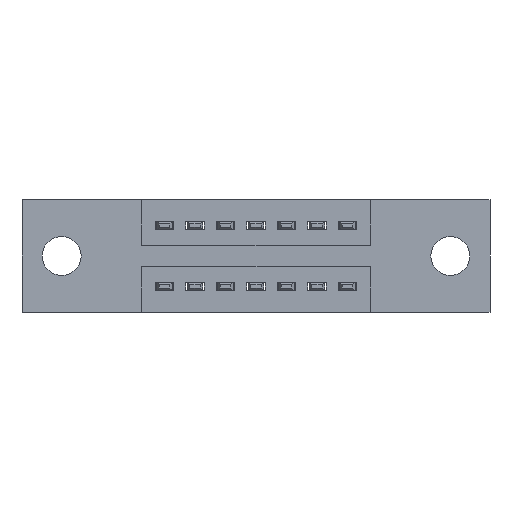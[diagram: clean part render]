
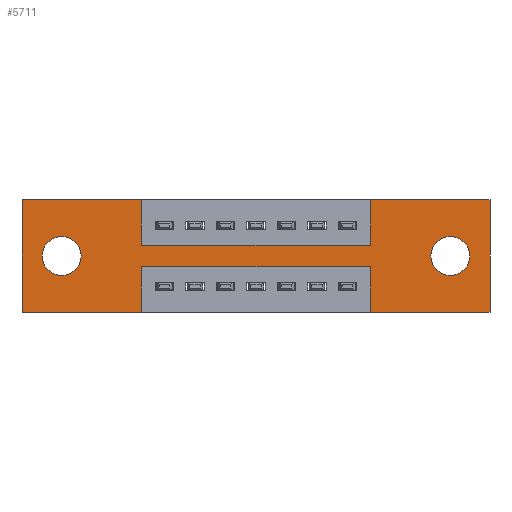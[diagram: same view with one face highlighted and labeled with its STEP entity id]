
A CAD part, front view. The second image highlights one B-rep face of the part: STEP entity #5711.
In plain terms, the highlighted planar face has unit normal (0, -1, 0).
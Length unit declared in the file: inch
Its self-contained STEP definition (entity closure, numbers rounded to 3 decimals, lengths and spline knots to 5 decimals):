
#54 = EDGE_CURVE ( 'NONE', #3700, #504, #7394, .T. ) ;
#79 = FACE_BOUND ( 'NONE', #6744, .T. ) ;
#148 = VECTOR ( 'NONE', #2319, 39.37008 ) ;
#348 = LINE ( 'NONE', #2535, #2153 ) ;
#473 = VERTEX_POINT ( 'NONE', #7672 ) ;
#504 = VERTEX_POINT ( 'NONE', #2349 ) ;
#685 = EDGE_CURVE ( 'NONE', #8767, #1796, #7384, .T. ) ;
#791 = DIRECTION ( 'NONE',  ( 1., 0., 0. ) ) ;
#833 = CIRCLE ( 'NONE', #9277, 0.064 ) ;
#880 = CIRCLE ( 'NONE', #2902, 0.064 ) ;
#932 = FACE_OUTER_BOUND ( 'NONE', #9668, .T. ) ;
#947 = CARTESIAN_POINT ( 'NONE',  ( 1.405, 0., -0.185 ) ) ;
#966 = DIRECTION ( 'NONE',  ( -1., 0., 0. ) ) ;
#981 = DIRECTION ( 'NONE',  ( 0., 1., 0. ) ) ;
#1031 = EDGE_CURVE ( 'NONE', #4648, #4432, #4263, .T. ) ;
#1047 = LINE ( 'NONE', #3530, #5956 ) ;
#1112 = LINE ( 'NONE', #1610, #9343 ) ;
#1265 = CARTESIAN_POINT ( 'NONE',  ( 0., 0., -0.37 ) ) ;
#1318 = AXIS2_PLACEMENT_3D ( 'NONE', #8120, #7399, #2808 ) ;
#1350 = CARTESIAN_POINT ( 'NONE',  ( 1.405, 0., -0.249 ) ) ;
#1355 = EDGE_CURVE ( 'NONE', #1935, #1695, #4728, .T. ) ;
#1462 = LINE ( 'NONE', #9288, #2197 ) ;
#1490 = VERTEX_POINT ( 'NONE', #4366 ) ;
#1610 = CARTESIAN_POINT ( 'NONE',  ( 1.1425, 0., -0.37 ) ) ;
#1665 = DIRECTION ( 'NONE',  ( 1., 0., 0. ) ) ;
#1684 = VERTEX_POINT ( 'NONE', #8054 ) ;
#1695 = VERTEX_POINT ( 'NONE', #8088 ) ;
#1796 = VERTEX_POINT ( 'NONE', #2870 ) ;
#1935 = VERTEX_POINT ( 'NONE', #3185 ) ;
#1985 = EDGE_CURVE ( 'NONE', #1796, #1935, #1112, .T. ) ;
#2035 = DIRECTION ( 'NONE',  ( 0., 0., -1. ) ) ;
#2130 = FACE_BOUND ( 'NONE', #6318, .T. ) ;
#2153 = VECTOR ( 'NONE', #4947, 39.37008 ) ;
#2197 = VECTOR ( 'NONE', #791, 39.37008 ) ;
#2272 = DIRECTION ( 'NONE',  ( 0., 1., 0. ) ) ;
#2319 = DIRECTION ( 'NONE',  ( 0., 0., 1. ) ) ;
#2349 = CARTESIAN_POINT ( 'NONE',  ( 1.405, 0., -0.121 ) ) ;
#2425 = DIRECTION ( 'NONE',  ( 0., 0., -1. ) ) ;
#2471 = CARTESIAN_POINT ( 'NONE',  ( 0.13, 0., -0.185 ) ) ;
#2478 = ORIENTED_EDGE ( 'NONE', *, *, #1985, .F. ) ;
#2535 = CARTESIAN_POINT ( 'NONE',  ( 1.1425, 0., 0. ) ) ;
#2577 = ORIENTED_EDGE ( 'NONE', *, *, #54, .T. ) ;
#2730 = DIRECTION ( 'NONE',  ( 0., 1., 0. ) ) ;
#2769 = VECTOR ( 'NONE', #2035, 39.37008 ) ;
#2808 = DIRECTION ( 'NONE',  ( 0., 0., -1. ) ) ;
#2814 = VECTOR ( 'NONE', #6021, 39.37008 ) ;
#2870 = CARTESIAN_POINT ( 'NONE',  ( 1.1425, 0., -0.37 ) ) ;
#2902 = AXIS2_PLACEMENT_3D ( 'NONE', #7319, #2730, #8102 ) ;
#2945 = CARTESIAN_POINT ( 'NONE',  ( 0.3925, 0., 0. ) ) ;
#2947 = LINE ( 'NONE', #1265, #6787 ) ;
#3185 = CARTESIAN_POINT ( 'NONE',  ( 1.1425, 0., -0.22 ) ) ;
#3530 = CARTESIAN_POINT ( 'NONE',  ( 0., 0., 0. ) ) ;
#3567 = EDGE_CURVE ( 'NONE', #473, #8945, #833, .T. ) ;
#3586 = VERTEX_POINT ( 'NONE', #5769 ) ;
#3681 = ORIENTED_EDGE ( 'NONE', *, *, #5395, .F. ) ;
#3700 = VERTEX_POINT ( 'NONE', #1350 ) ;
#3935 = CARTESIAN_POINT ( 'NONE',  ( 0.3925, 0., -0.22 ) ) ;
#4042 = CARTESIAN_POINT ( 'NONE',  ( 0., 0., -0.37 ) ) ;
#4152 = EDGE_CURVE ( 'NONE', #3586, #4873, #348, .T. ) ;
#4258 = CARTESIAN_POINT ( 'NONE',  ( 1.535, 0., 0. ) ) ;
#4263 = LINE ( 'NONE', #9400, #148 ) ;
#4309 = VECTOR ( 'NONE', #1665, 39.37008 ) ;
#4366 = CARTESIAN_POINT ( 'NONE',  ( 0.3925, 0., -0.15 ) ) ;
#4381 = EDGE_CURVE ( 'NONE', #1695, #8829, #4810, .T. ) ;
#4431 = CARTESIAN_POINT ( 'NONE',  ( 0., 0., -0.37 ) ) ;
#4432 = VERTEX_POINT ( 'NONE', #7391 ) ;
#4583 = ORIENTED_EDGE ( 'NONE', *, *, #4152, .F. ) ;
#4648 = VERTEX_POINT ( 'NONE', #4431 ) ;
#4728 = LINE ( 'NONE', #3935, #8218 ) ;
#4747 = CARTESIAN_POINT ( 'NONE',  ( 0.3925, 0., -0.15 ) ) ;
#4810 = LINE ( 'NONE', #5676, #2769 ) ;
#4873 = VERTEX_POINT ( 'NONE', #8543 ) ;
#4947 = DIRECTION ( 'NONE',  ( 0., 0., 1. ) ) ;
#5012 = ORIENTED_EDGE ( 'NONE', *, *, #9839, .T. ) ;
#5086 = CARTESIAN_POINT ( 'NONE',  ( 0.3925, 0., -0.37 ) ) ;
#5132 = ORIENTED_EDGE ( 'NONE', *, *, #1031, .F. ) ;
#5139 = AXIS2_PLACEMENT_3D ( 'NONE', #5803, #2272, #5225 ) ;
#5218 = CARTESIAN_POINT ( 'NONE',  ( 1.535, 0., 0. ) ) ;
#5225 = DIRECTION ( 'NONE',  ( 0., 0., -1. ) ) ;
#5279 = ORIENTED_EDGE ( 'NONE', *, *, #4381, .F. ) ;
#5284 = ORIENTED_EDGE ( 'NONE', *, *, #6078, .F. ) ;
#5395 = EDGE_CURVE ( 'NONE', #1490, #3586, #8045, .T. ) ;
#5551 = VERTEX_POINT ( 'NONE', #4258 ) ;
#5676 = CARTESIAN_POINT ( 'NONE',  ( 0.3925, 0., -0.37 ) ) ;
#5711 = ADVANCED_FACE ( 'NONE', ( #2130, #79, #932 ), #5836, .T. ) ;
#5769 = CARTESIAN_POINT ( 'NONE',  ( 1.1425, 0., -0.15 ) ) ;
#5803 = CARTESIAN_POINT ( 'NONE',  ( 1.405, 0., -0.185 ) ) ;
#5836 = PLANE ( 'NONE',  #1318 ) ;
#5927 = DIRECTION ( 'NONE',  ( 0., 0., -1. ) ) ;
#5956 = VECTOR ( 'NONE', #9735, 39.37008 ) ;
#5990 = ORIENTED_EDGE ( 'NONE', *, *, #3567, .T. ) ;
#6021 = DIRECTION ( 'NONE',  ( 0., 0., -1. ) ) ;
#6078 = EDGE_CURVE ( 'NONE', #4873, #5551, #1047, .T. ) ;
#6120 = ORIENTED_EDGE ( 'NONE', *, *, #8074, .F. ) ;
#6236 = ORIENTED_EDGE ( 'NONE', *, *, #6897, .F. ) ;
#6318 = EDGE_LOOP ( 'NONE', ( #9372, #2577 ) ) ;
#6438 = CARTESIAN_POINT ( 'NONE',  ( 1.535, 0., -0.37 ) ) ;
#6656 = EDGE_CURVE ( 'NONE', #504, #3700, #8640, .T. ) ;
#6744 = EDGE_LOOP ( 'NONE', ( #5012, #5990 ) ) ;
#6787 = VECTOR ( 'NONE', #7158, 39.37008 ) ;
#6856 = DIRECTION ( 'NONE',  ( 0., 0., 1. ) ) ;
#6897 = EDGE_CURVE ( 'NONE', #8829, #4648, #2947, .T. ) ;
#7022 = DIRECTION ( 'NONE',  ( -1., 0., 0. ) ) ;
#7158 = DIRECTION ( 'NONE',  ( -1., 0., 0. ) ) ;
#7276 = VECTOR ( 'NONE', #966, 39.37008 ) ;
#7319 = CARTESIAN_POINT ( 'NONE',  ( 0.13, 0., -0.185 ) ) ;
#7384 = LINE ( 'NONE', #4042, #7276 ) ;
#7391 = CARTESIAN_POINT ( 'NONE',  ( 0., 0., 0. ) ) ;
#7394 = CIRCLE ( 'NONE', #5139, 0.064 ) ;
#7399 = DIRECTION ( 'NONE',  ( 0., -1., 0. ) ) ;
#7646 = EDGE_CURVE ( 'NONE', #5551, #8767, #8004, .T. ) ;
#7672 = CARTESIAN_POINT ( 'NONE',  ( 0.13, 0., -0.249 ) ) ;
#7729 = ORIENTED_EDGE ( 'NONE', *, *, #685, .F. ) ;
#7946 = EDGE_CURVE ( 'NONE', #4432, #1684, #1462, .T. ) ;
#8004 = LINE ( 'NONE', #5218, #9351 ) ;
#8045 = LINE ( 'NONE', #4747, #4309 ) ;
#8054 = CARTESIAN_POINT ( 'NONE',  ( 0.3925, 0., 0. ) ) ;
#8074 = EDGE_CURVE ( 'NONE', #1684, #1490, #8989, .T. ) ;
#8088 = CARTESIAN_POINT ( 'NONE',  ( 0.3925, 0., -0.22 ) ) ;
#8090 = ORIENTED_EDGE ( 'NONE', *, *, #1355, .F. ) ;
#8102 = DIRECTION ( 'NONE',  ( 0., 0., 1. ) ) ;
#8120 = CARTESIAN_POINT ( 'NONE',  ( 0., 0., -0.37 ) ) ;
#8214 = ORIENTED_EDGE ( 'NONE', *, *, #7646, .F. ) ;
#8218 = VECTOR ( 'NONE', #7022, 39.37008 ) ;
#8543 = CARTESIAN_POINT ( 'NONE',  ( 1.1425, 0., 0. ) ) ;
#8640 = CIRCLE ( 'NONE', #9577, 0.064 ) ;
#8767 = VERTEX_POINT ( 'NONE', #6438 ) ;
#8808 = ORIENTED_EDGE ( 'NONE', *, *, #7946, .F. ) ;
#8829 = VERTEX_POINT ( 'NONE', #5086 ) ;
#8945 = VERTEX_POINT ( 'NONE', #9096 ) ;
#8989 = LINE ( 'NONE', #2945, #2814 ) ;
#9096 = CARTESIAN_POINT ( 'NONE',  ( 0.13, 0., -0.121 ) ) ;
#9277 = AXIS2_PLACEMENT_3D ( 'NONE', #2471, #9405, #9520 ) ;
#9288 = CARTESIAN_POINT ( 'NONE',  ( 0., 0., 0. ) ) ;
#9343 = VECTOR ( 'NONE', #6856, 39.37008 ) ;
#9351 = VECTOR ( 'NONE', #5927, 39.37008 ) ;
#9372 = ORIENTED_EDGE ( 'NONE', *, *, #6656, .T. ) ;
#9400 = CARTESIAN_POINT ( 'NONE',  ( 0., 0., 0. ) ) ;
#9405 = DIRECTION ( 'NONE',  ( 0., 1., 0. ) ) ;
#9520 = DIRECTION ( 'NONE',  ( 0., 0., 1. ) ) ;
#9577 = AXIS2_PLACEMENT_3D ( 'NONE', #947, #981, #2425 ) ;
#9668 = EDGE_LOOP ( 'NONE', ( #5279, #8090, #2478, #7729, #8214, #5284, #4583, #3681, #6120, #8808, #5132, #6236 ) ) ;
#9735 = DIRECTION ( 'NONE',  ( 1., 0., 0. ) ) ;
#9839 = EDGE_CURVE ( 'NONE', #8945, #473, #880, .T. ) ;
